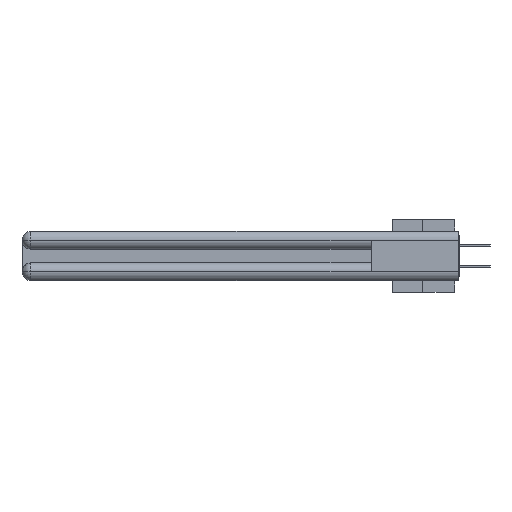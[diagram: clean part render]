
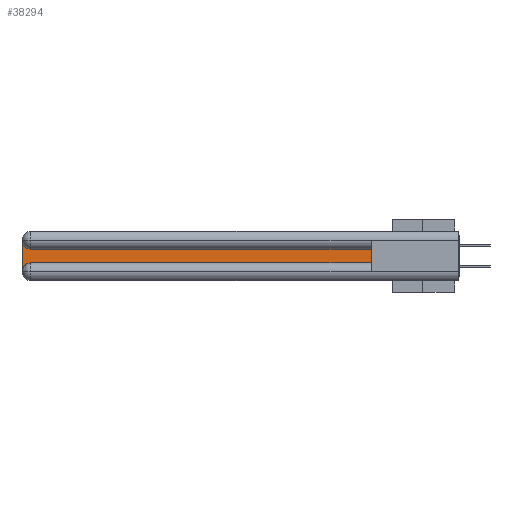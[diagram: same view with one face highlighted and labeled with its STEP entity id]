
A CAD part, left-side view. The second image highlights one B-rep face of the part: STEP entity #38294.
In plain terms, the highlighted planar face has unit normal (-1, 0, 0).
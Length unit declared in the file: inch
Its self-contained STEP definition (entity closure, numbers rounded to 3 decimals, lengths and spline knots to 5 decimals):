
#385 = VERTEX_POINT ( 'NONE', #29449 ) ;
#2556 = EDGE_CURVE ( 'NONE', #385, #8901, #3746, .T. ) ;
#3154 = VECTOR ( 'NONE', #24716, 39.37008 ) ;
#3746 = CIRCLE ( 'NONE', #10552, 0.06 ) ;
#4007 = CARTESIAN_POINT ( 'NONE',  ( 0.075, 0.6, -0.2175 ) ) ;
#4670 = AXIS2_PLACEMENT_3D ( 'NONE', #11168, #7916, #38538 ) ;
#7284 = ORIENTED_EDGE ( 'NONE', *, *, #10120, .T. ) ;
#7916 = DIRECTION ( 'NONE',  ( 1., 0., 0. ) ) ;
#8700 = PLANE ( 'NONE',  #25293 ) ;
#8901 = VERTEX_POINT ( 'NONE', #20855 ) ;
#9866 = CARTESIAN_POINT ( 'NONE',  ( 0.075, 0.6, -0.2175 ) ) ;
#10120 = EDGE_CURVE ( 'NONE', #36454, #385, #30176, .T. ) ;
#10552 = AXIS2_PLACEMENT_3D ( 'NONE', #24770, #41842, #21445 ) ;
#10585 = ORIENTED_EDGE ( 'NONE', *, *, #2556, .T. ) ;
#11168 = CARTESIAN_POINT ( 'NONE',  ( 0.075, 2.94, -0.2775 ) ) ;
#12742 = LINE ( 'NONE', #4007, #3154 ) ;
#15801 = DIRECTION ( 'NONE',  ( 1., 0., 0. ) ) ;
#16177 = CARTESIAN_POINT ( 'NONE',  ( 0.075, 3., -0.2175 ) ) ;
#16747 = DIRECTION ( 'NONE',  ( 0., 0., -1. ) ) ;
#16999 = DIRECTION ( 'NONE',  ( 0., -1., 0. ) ) ;
#17410 = VECTOR ( 'NONE', #39987, 39.37008 ) ;
#20015 = VERTEX_POINT ( 'NONE', #41053 ) ;
#20035 = CARTESIAN_POINT ( 'NONE',  ( 0.075, 0.6, -0.1225 ) ) ;
#20129 = CARTESIAN_POINT ( 'NONE',  ( 0.075, 2.94, -0.2175 ) ) ;
#20855 = CARTESIAN_POINT ( 'NONE',  ( 0.075, 3., -0.0625 ) ) ;
#20993 = ORIENTED_EDGE ( 'NONE', *, *, #36990, .T. ) ;
#21445 = DIRECTION ( 'NONE',  ( 0., 0., -1. ) ) ;
#22643 = DIRECTION ( 'NONE',  ( 0., 0., -1. ) ) ;
#23132 = EDGE_CURVE ( 'NONE', #23209, #20015, #29458, .T. ) ;
#23209 = VERTEX_POINT ( 'NONE', #20129 ) ;
#23671 = CARTESIAN_POINT ( 'NONE',  ( 0.075, 0.6, -0.1225 ) ) ;
#23816 = CARTESIAN_POINT ( 'NONE',  ( 0.075, 3., -0.2775 ) ) ;
#24716 = DIRECTION ( 'NONE',  ( 0., 0., 1. ) ) ;
#24770 = CARTESIAN_POINT ( 'NONE',  ( 0.075, 2.94, -0.0625 ) ) ;
#25293 = AXIS2_PLACEMENT_3D ( 'NONE', #36173, #15801, #22643 ) ;
#25907 = EDGE_CURVE ( 'NONE', #33685, #23209, #31654, .T. ) ;
#26594 = EDGE_LOOP ( 'NONE', ( #7284, #10585, #28869, #26596, #32507, #20993 ) ) ;
#26596 = ORIENTED_EDGE ( 'NONE', *, *, #25907, .T. ) ;
#28869 = ORIENTED_EDGE ( 'NONE', *, *, #30254, .T. ) ;
#29449 = CARTESIAN_POINT ( 'NONE',  ( 0.075, 2.94, -0.1225 ) ) ;
#29458 = LINE ( 'NONE', #9866, #31566 ) ;
#30176 = LINE ( 'NONE', #20035, #17410 ) ;
#30254 = EDGE_CURVE ( 'NONE', #8901, #33685, #37456, .T. ) ;
#30733 = FACE_OUTER_BOUND ( 'NONE', #26594, .T. ) ;
#31566 = VECTOR ( 'NONE', #16999, 39.37008 ) ;
#31654 = CIRCLE ( 'NONE', #4670, 0.06 ) ;
#32507 = ORIENTED_EDGE ( 'NONE', *, *, #23132, .T. ) ;
#32702 = VECTOR ( 'NONE', #16747, 39.37008 ) ;
#33685 = VERTEX_POINT ( 'NONE', #23816 ) ;
#36173 = CARTESIAN_POINT ( 'NONE',  ( 0.075, 3., -0.1225 ) ) ;
#36454 = VERTEX_POINT ( 'NONE', #23671 ) ;
#36990 = EDGE_CURVE ( 'NONE', #20015, #36454, #12742, .T. ) ;
#37456 = LINE ( 'NONE', #16177, #32702 ) ;
#38294 = ADVANCED_FACE ( 'NONE', ( #30733 ), #8700, .F. ) ;
#38538 = DIRECTION ( 'NONE',  ( 0., 0., -1. ) ) ;
#39987 = DIRECTION ( 'NONE',  ( 0., 1., 0. ) ) ;
#41053 = CARTESIAN_POINT ( 'NONE',  ( 0.075, 0.6, -0.2175 ) ) ;
#41842 = DIRECTION ( 'NONE',  ( 1., 0., 0. ) ) ;
